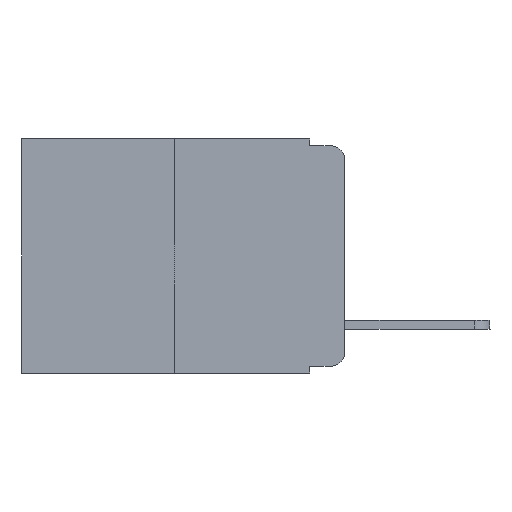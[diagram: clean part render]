
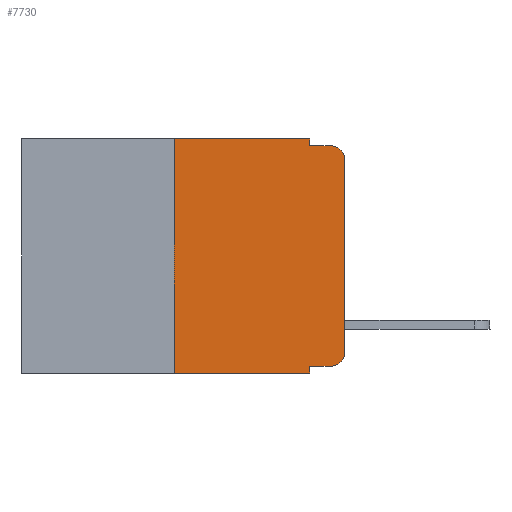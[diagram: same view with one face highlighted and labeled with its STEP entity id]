
A CAD part, left-side view. The second image highlights one B-rep face of the part: STEP entity #7730.
In plain terms, the highlighted planar face has unit normal (-1, 0, 0).
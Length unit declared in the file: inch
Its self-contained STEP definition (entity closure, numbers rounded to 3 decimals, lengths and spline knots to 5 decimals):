
#538 = ORIENTED_EDGE ( 'NONE', *, *, #1949, .F. ) ;
#1065 = ORIENTED_EDGE ( 'NONE', *, *, #6985, .F. ) ;
#1450 = VECTOR ( 'NONE', #13345, 39.37008 ) ;
#1949 = EDGE_CURVE ( 'NONE', #8518, #11153, #11711, .T. ) ;
#2186 = CARTESIAN_POINT ( 'NONE',  ( 0., 0.051, -0.333 ) ) ;
#2364 = CARTESIAN_POINT ( 'NONE',  ( 0., 0.051, -0.333 ) ) ;
#2407 = ORIENTED_EDGE ( 'NONE', *, *, #5768, .F. ) ;
#2411 = ORIENTED_EDGE ( 'NONE', *, *, #7712, .T. ) ;
#2778 = CARTESIAN_POINT ( 'NONE',  ( 0., 0.051, -0.01 ) ) ;
#2881 = VECTOR ( 'NONE', #10924, 39.37008 ) ;
#3132 = CARTESIAN_POINT ( 'NONE',  ( 0., 0.473, 0. ) ) ;
#3340 = LINE ( 'NONE', #4381, #7560 ) ;
#3366 = LINE ( 'NONE', #12090, #1450 ) ;
#3532 = DIRECTION ( 'NONE',  ( 0., -1., 0. ) ) ;
#3628 = VERTEX_POINT ( 'NONE', #7567 ) ;
#3724 = EDGE_CURVE ( 'NONE', #11153, #14149, #8571, .T. ) ;
#4190 = EDGE_CURVE ( 'NONE', #3628, #11322, #4785, .T. ) ;
#4381 = CARTESIAN_POINT ( 'NONE',  ( 0., 0., 0. ) ) ;
#4527 = CARTESIAN_POINT ( 'NONE',  ( 0., 0.473, 0. ) ) ;
#4597 = AXIS2_PLACEMENT_3D ( 'NONE', #13063, #7393, #12997 ) ;
#4725 = VERTEX_POINT ( 'NONE', #8360 ) ;
#4785 = LINE ( 'NONE', #9051, #5683 ) ;
#5373 = AXIS2_PLACEMENT_3D ( 'NONE', #14197, #13040, #12968 ) ;
#5652 = CARTESIAN_POINT ( 'NONE',  ( 0., 0.02, -0.01 ) ) ;
#5683 = VECTOR ( 'NONE', #3532, 39.37008 ) ;
#5706 = VECTOR ( 'NONE', #10907, 39.37008 ) ;
#5768 = EDGE_CURVE ( 'NONE', #3628, #11295, #3366, .T. ) ;
#5833 = ORIENTED_EDGE ( 'NONE', *, *, #3724, .F. ) ;
#6192 = EDGE_CURVE ( 'NONE', #11295, #8518, #12955, .T. ) ;
#6469 = CARTESIAN_POINT ( 'NONE',  ( 0., 0.051, -0.343 ) ) ;
#6718 = FACE_OUTER_BOUND ( 'NONE', #12899, .T. ) ;
#6790 = VERTEX_POINT ( 'NONE', #7845 ) ;
#6985 = EDGE_CURVE ( 'NONE', #9310, #11322, #10799, .T. ) ;
#7359 = DIRECTION ( 'NONE',  ( 0., 0., -1. ) ) ;
#7393 = DIRECTION ( 'NONE',  ( -1., 0., 0. ) ) ;
#7560 = VECTOR ( 'NONE', #13536, 39.37008 ) ;
#7562 = EDGE_CURVE ( 'NONE', #9310, #10212, #7675, .T. ) ;
#7567 = CARTESIAN_POINT ( 'NONE',  ( 0., 0.25, -0.343 ) ) ;
#7675 = LINE ( 'NONE', #2186, #2881 ) ;
#7696 = VECTOR ( 'NONE', #13091, 39.37008 ) ;
#7712 = EDGE_CURVE ( 'NONE', #4725, #6790, #3340, .T. ) ;
#7730 = ADVANCED_FACE ( 'NONE', ( #6718 ), #9869, .F. ) ;
#7845 = CARTESIAN_POINT ( 'NONE',  ( 0., 0., -0.03 ) ) ;
#8098 = ORIENTED_EDGE ( 'NONE', *, *, #4190, .T. ) ;
#8360 = CARTESIAN_POINT ( 'NONE',  ( 0., 0., -0.313 ) ) ;
#8518 = VERTEX_POINT ( 'NONE', #11216 ) ;
#8571 = LINE ( 'NONE', #8641, #7696 ) ;
#8641 = CARTESIAN_POINT ( 'NONE',  ( 0., 0.051, -0.01 ) ) ;
#9046 = ORIENTED_EDGE ( 'NONE', *, *, #14040, .T. ) ;
#9051 = CARTESIAN_POINT ( 'NONE',  ( 0., 0.473, -0.343 ) ) ;
#9310 = VERTEX_POINT ( 'NONE', #2364 ) ;
#9590 = EDGE_CURVE ( 'NONE', #10212, #4725, #12699, .T. ) ;
#9608 = VECTOR ( 'NONE', #11748, 39.37008 ) ;
#9668 = ORIENTED_EDGE ( 'NONE', *, *, #6192, .F. ) ;
#9869 = PLANE ( 'NONE',  #13371 ) ;
#10212 = VERTEX_POINT ( 'NONE', #11059 ) ;
#10799 = LINE ( 'NONE', #13135, #9608 ) ;
#10803 = VECTOR ( 'NONE', #7359, 39.37008 ) ;
#10907 = DIRECTION ( 'NONE',  ( 0., -1., 0. ) ) ;
#10924 = DIRECTION ( 'NONE',  ( 0., -1., 0. ) ) ;
#11059 = CARTESIAN_POINT ( 'NONE',  ( 0., 0.02, -0.333 ) ) ;
#11153 = VERTEX_POINT ( 'NONE', #2778 ) ;
#11216 = CARTESIAN_POINT ( 'NONE',  ( 0., 0.051, 0. ) ) ;
#11233 = ORIENTED_EDGE ( 'NONE', *, *, #7562, .T. ) ;
#11295 = VERTEX_POINT ( 'NONE', #13928 ) ;
#11322 = VERTEX_POINT ( 'NONE', #6469 ) ;
#11571 = CARTESIAN_POINT ( 'NONE',  ( 0., 0.051, 0. ) ) ;
#11711 = LINE ( 'NONE', #11571, #10803 ) ;
#11748 = DIRECTION ( 'NONE',  ( 0., 0., -1. ) ) ;
#11988 = ORIENTED_EDGE ( 'NONE', *, *, #9590, .T. ) ;
#12090 = CARTESIAN_POINT ( 'NONE',  ( 0., 0.25, 0. ) ) ;
#12543 = CIRCLE ( 'NONE', #5373, 0.02 ) ;
#12699 = CIRCLE ( 'NONE', #4597, 0.02 ) ;
#12899 = EDGE_LOOP ( 'NONE', ( #2411, #9046, #5833, #538, #9668, #2407, #8098, #1065, #11233, #11988 ) ) ;
#12955 = LINE ( 'NONE', #3132, #5706 ) ;
#12968 = DIRECTION ( 'NONE',  ( 0., 0., -1. ) ) ;
#12997 = DIRECTION ( 'NONE',  ( 0., 0., -1. ) ) ;
#13040 = DIRECTION ( 'NONE',  ( -1., 0., 0. ) ) ;
#13063 = CARTESIAN_POINT ( 'NONE',  ( 0., 0.02, -0.313 ) ) ;
#13091 = DIRECTION ( 'NONE',  ( 0., -1., 0. ) ) ;
#13135 = CARTESIAN_POINT ( 'NONE',  ( 0., 0.051, 0. ) ) ;
#13316 = DIRECTION ( 'NONE',  ( 1., 0., 0. ) ) ;
#13345 = DIRECTION ( 'NONE',  ( 0., 0., 1. ) ) ;
#13371 = AXIS2_PLACEMENT_3D ( 'NONE', #4527, #13316, #14323 ) ;
#13536 = DIRECTION ( 'NONE',  ( 0., 0., 1. ) ) ;
#13928 = CARTESIAN_POINT ( 'NONE',  ( 0., 0.25, 0. ) ) ;
#14040 = EDGE_CURVE ( 'NONE', #6790, #14149, #12543, .T. ) ;
#14149 = VERTEX_POINT ( 'NONE', #5652 ) ;
#14197 = CARTESIAN_POINT ( 'NONE',  ( 0., 0.02, -0.03 ) ) ;
#14323 = DIRECTION ( 'NONE',  ( 0., 0., -1. ) ) ;
